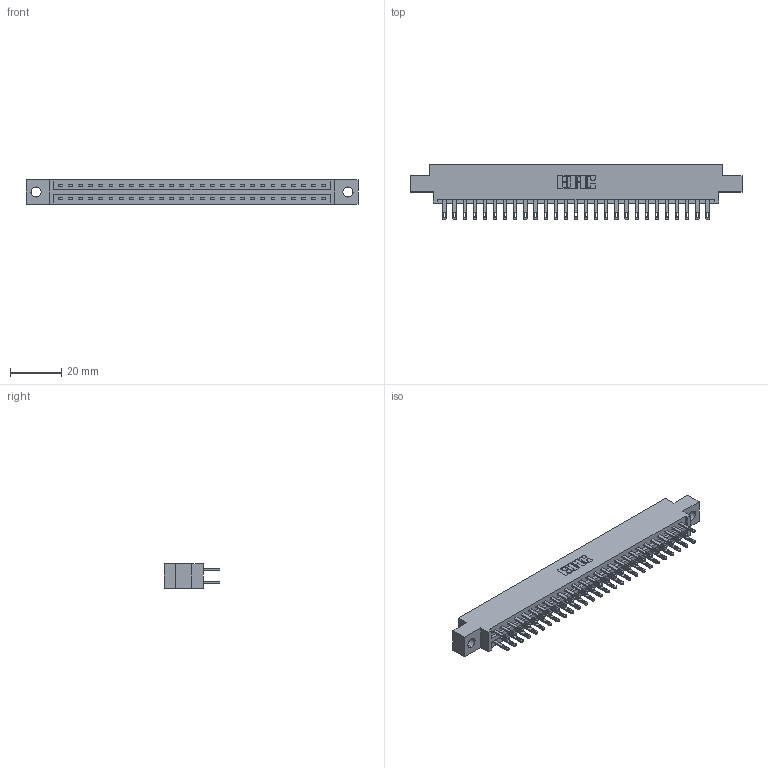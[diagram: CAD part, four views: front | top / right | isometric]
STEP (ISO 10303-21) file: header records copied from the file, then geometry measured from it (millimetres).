
FILE_DESCRIPTION (( 'STEP AP203' ), '1' );
FILE_NAME ('337-054-500-804.STEP', '2018-08-10T00:01:29', ( '' ), ( '' ), 'SwSTEP 2.0', 'SolidWorks 2016', '' );
FILE_SCHEMA (( 'CONFIG_CONTROL_DESIGN' ));
Length unit declared in the file: inch
Products named in the file (3): 337 Part_0.170 Offset - 0.156 Dia-TH; 345-292-001_345-293-100; 337-054-500-804
Assembly tree (55 placements, depth 2):
  337-054-500-804
    337 Part_0.170 Offset - 0.156 Dia-TH
    345-292-001_345-293-100  x54
Bounding box: 130 x 21.85 x 9.4 mm (x, y, z)
Volume: 13460.1 mm3; surface area: 15575.4 mm2
Topology: 55 solids, 55 shells, 2818 faces, 8585 edges, 5722 vertices
Faces by surface type: plane 1802, cylinder 1016
Entity records: 22939 total; most frequent: CARTESIAN_POINT 3878, ORIENTED_EDGE 3814, DIRECTION 3327, EDGE_CURVE 1907, LINE 1775, VECTOR 1775, VERTEX_POINT 1270, AXIS2_PLACEMENT_3D 776
